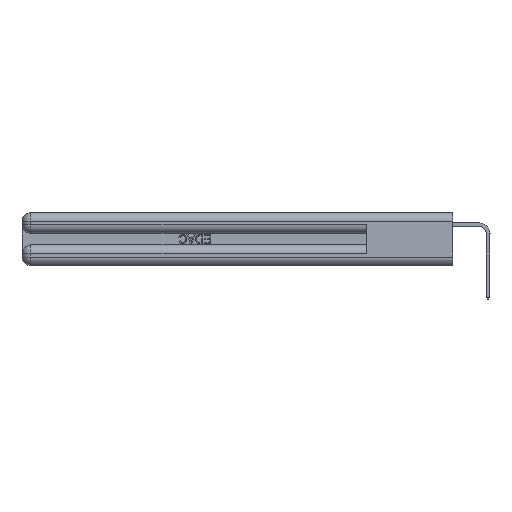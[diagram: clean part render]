
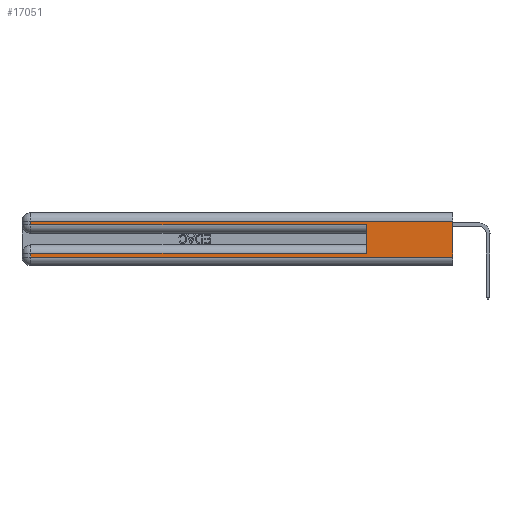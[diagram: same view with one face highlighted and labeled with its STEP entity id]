
A CAD part, left-side view. The second image highlights one B-rep face of the part: STEP entity #17051.
In plain terms, the highlighted planar face has unit normal (-1, 0, 0).
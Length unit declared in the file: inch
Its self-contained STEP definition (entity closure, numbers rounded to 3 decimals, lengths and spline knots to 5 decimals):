
#325 = DIRECTION ( 'NONE',  ( 0., 0., -1. ) ) ;
#1344 = DIRECTION ( 'NONE',  ( 0., 1., 0. ) ) ;
#1837 = VECTOR ( 'NONE', #28523, 39.37008 ) ;
#1854 = LINE ( 'NONE', #28563, #20870 ) ;
#1901 = DIRECTION ( 'NONE',  ( 0., 0., -1. ) ) ;
#1915 = EDGE_CURVE ( 'NONE', #13714, #19796, #1854, .T. ) ;
#2258 = CARTESIAN_POINT ( 'NONE',  ( 0., 2.94, 0.31 ) ) ;
#3138 = CARTESIAN_POINT ( 'NONE',  ( 0., 2.94, 0.085 ) ) ;
#3589 = EDGE_LOOP ( 'NONE', ( #43268, #32980, #38107, #22759, #7503, #13251, #11024, #39198 ) ) ;
#4222 = LINE ( 'NONE', #13358, #1837 ) ;
#4527 = CARTESIAN_POINT ( 'NONE',  ( 0., 0.6, 0.085 ) ) ;
#5722 = CARTESIAN_POINT ( 'NONE',  ( 0., 0.6, 0.285 ) ) ;
#7503 = ORIENTED_EDGE ( 'NONE', *, *, #17194, .F. ) ;
#8653 = EDGE_CURVE ( 'NONE', #9627, #10911, #25738, .T. ) ;
#9006 = VERTEX_POINT ( 'NONE', #5722 ) ;
#9097 = LINE ( 'NONE', #37639, #28002 ) ;
#9627 = VERTEX_POINT ( 'NONE', #43781 ) ;
#10911 = VERTEX_POINT ( 'NONE', #21959 ) ;
#11024 = ORIENTED_EDGE ( 'NONE', *, *, #27304, .T. ) ;
#11148 = DIRECTION ( 'NONE',  ( 0., 0., -1. ) ) ;
#11465 = VERTEX_POINT ( 'NONE', #3138 ) ;
#12153 = EDGE_CURVE ( 'NONE', #19796, #9006, #33719, .T. ) ;
#13251 = ORIENTED_EDGE ( 'NONE', *, *, #37541, .T. ) ;
#13358 = CARTESIAN_POINT ( 'NONE',  ( 0., 0., 0.085 ) ) ;
#13714 = VERTEX_POINT ( 'NONE', #2258 ) ;
#14216 = DIRECTION ( 'NONE',  ( 0., 0., 1. ) ) ;
#15691 = VECTOR ( 'NONE', #33739, 39.37008 ) ;
#17007 = PLANE ( 'NONE',  #22042 ) ;
#17051 = ADVANCED_FACE ( 'NONE', ( #29104 ), #17007, .F. ) ;
#17194 = EDGE_CURVE ( 'NONE', #19251, #9006, #42164, .T. ) ;
#19251 = VERTEX_POINT ( 'NONE', #4527 ) ;
#19796 = VERTEX_POINT ( 'NONE', #43736 ) ;
#20669 = EDGE_CURVE ( 'NONE', #35021, #10911, #29024, .T. ) ;
#20870 = VECTOR ( 'NONE', #32399, 39.37008 ) ;
#21959 = CARTESIAN_POINT ( 'NONE',  ( 0., 0., 0.06 ) ) ;
#21996 = DIRECTION ( 'NONE',  ( 0., -1., 0. ) ) ;
#22042 = AXIS2_PLACEMENT_3D ( 'NONE', #47383, #24623, #1901 ) ;
#22759 = ORIENTED_EDGE ( 'NONE', *, *, #12153, .T. ) ;
#23081 = CARTESIAN_POINT ( 'NONE',  ( 0., 0., 0.37 ) ) ;
#24089 = CARTESIAN_POINT ( 'NONE',  ( 0., 0., 0.31 ) ) ;
#24623 = DIRECTION ( 'NONE',  ( 1., 0., 0. ) ) ;
#24815 = VECTOR ( 'NONE', #21996, 39.37008 ) ;
#25738 = LINE ( 'NONE', #45225, #15691 ) ;
#27304 = EDGE_CURVE ( 'NONE', #11465, #9627, #9097, .T. ) ;
#28002 = VECTOR ( 'NONE', #11148, 39.37008 ) ;
#28523 = DIRECTION ( 'NONE',  ( 0., 1., 0. ) ) ;
#28563 = CARTESIAN_POINT ( 'NONE',  ( 0., 2.94, 0.37 ) ) ;
#29024 = LINE ( 'NONE', #23081, #47480 ) ;
#29104 = FACE_OUTER_BOUND ( 'NONE', #3589, .T. ) ;
#31304 = LINE ( 'NONE', #24089, #32511 ) ;
#32399 = DIRECTION ( 'NONE',  ( 0., 0., -1. ) ) ;
#32511 = VECTOR ( 'NONE', #1344, 39.37008 ) ;
#32980 = ORIENTED_EDGE ( 'NONE', *, *, #48679, .T. ) ;
#33259 = VECTOR ( 'NONE', #14216, 39.37008 ) ;
#33719 = LINE ( 'NONE', #48543, #24815 ) ;
#33739 = DIRECTION ( 'NONE',  ( 0., -1., 0. ) ) ;
#35021 = VERTEX_POINT ( 'NONE', #47514 ) ;
#36907 = CARTESIAN_POINT ( 'NONE',  ( 0., 0.6, 0.145 ) ) ;
#37541 = EDGE_CURVE ( 'NONE', #19251, #11465, #4222, .T. ) ;
#37639 = CARTESIAN_POINT ( 'NONE',  ( 0., 2.94, 0.37 ) ) ;
#38107 = ORIENTED_EDGE ( 'NONE', *, *, #1915, .T. ) ;
#39198 = ORIENTED_EDGE ( 'NONE', *, *, #8653, .T. ) ;
#42164 = LINE ( 'NONE', #36907, #33259 ) ;
#43268 = ORIENTED_EDGE ( 'NONE', *, *, #20669, .F. ) ;
#43736 = CARTESIAN_POINT ( 'NONE',  ( 0., 2.94, 0.285 ) ) ;
#43781 = CARTESIAN_POINT ( 'NONE',  ( 0., 2.94, 0.06 ) ) ;
#45225 = CARTESIAN_POINT ( 'NONE',  ( 0., 0., 0.06 ) ) ;
#47383 = CARTESIAN_POINT ( 'NONE',  ( 0., 0., 0.37 ) ) ;
#47480 = VECTOR ( 'NONE', #325, 39.37008 ) ;
#47514 = CARTESIAN_POINT ( 'NONE',  ( 0., 0., 0.31 ) ) ;
#48543 = CARTESIAN_POINT ( 'NONE',  ( 0., 0., 0.285 ) ) ;
#48679 = EDGE_CURVE ( 'NONE', #35021, #13714, #31304, .T. ) ;
